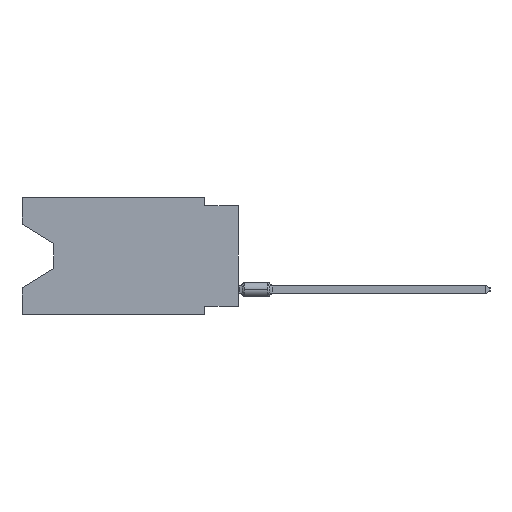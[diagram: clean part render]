
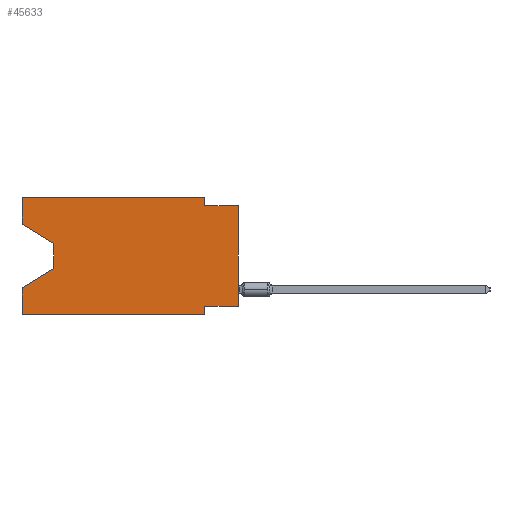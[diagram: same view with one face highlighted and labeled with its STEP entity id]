
A CAD part, left-side view. The second image highlights one B-rep face of the part: STEP entity #45633.
In plain terms, the highlighted planar face has unit normal (-1, 0, 0).
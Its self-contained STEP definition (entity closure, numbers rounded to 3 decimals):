
#1203 = LINE ( 'NONE', #77427, #64038 ) ;
#1259 = EDGE_CURVE ( 'NONE', #56919, #22937, #66565, .T. ) ;
#1292 = CARTESIAN_POINT ( 'NONE',  ( 0., 13.97, -3.505 ) ) ;
#2321 = CARTESIAN_POINT ( 'NONE',  ( 0., 2.54, -8.255 ) ) ;
#2335 = CARTESIAN_POINT ( 'NONE',  ( 0., 16.383, -2.038 ) ) ;
#3338 = CARTESIAN_POINT ( 'NONE',  ( 0., 16.383, -2.038 ) ) ;
#3871 = PLANE ( 'NONE',  #79965 ) ;
#4472 = LINE ( 'NONE', #100131, #5257 ) ;
#5257 = VECTOR ( 'NONE', #88839, 1000. ) ;
#7312 = CARTESIAN_POINT ( 'NONE',  ( 0., 13.97, -3.505 ) ) ;
#7677 = CARTESIAN_POINT ( 'NONE',  ( 0., 0., -8.255 ) ) ;
#10876 = EDGE_CURVE ( 'NONE', #61296, #36003, #45650, .T. ) ;
#11784 = VECTOR ( 'NONE', #57175, 1000. ) ;
#12044 = VECTOR ( 'NONE', #87257, 1000. ) ;
#12978 = VERTEX_POINT ( 'NONE', #103977 ) ;
#13083 = LINE ( 'NONE', #3338, #11784 ) ;
#14751 = VECTOR ( 'NONE', #19941, 1000. ) ;
#15023 = CARTESIAN_POINT ( 'NONE',  ( 0., 13.97, -5.385 ) ) ;
#15088 = EDGE_CURVE ( 'NONE', #56919, #23978, #79063, .T. ) ;
#15566 = CARTESIAN_POINT ( 'NONE',  ( 0., 0., 0. ) ) ;
#16709 = LINE ( 'NONE', #26407, #110979 ) ;
#16798 = CARTESIAN_POINT ( 'NONE',  ( 0., 2.54, -0.635 ) ) ;
#17405 = VECTOR ( 'NONE', #88220, 1000. ) ;
#17586 = EDGE_CURVE ( 'NONE', #28885, #36003, #4472, .T. ) ;
#19941 = DIRECTION ( 'NONE',  ( 0., 0., -1. ) ) ;
#21270 = VERTEX_POINT ( 'NONE', #2335 ) ;
#21811 = ORIENTED_EDGE ( 'NONE', *, *, #25461, .F. ) ;
#22937 = VERTEX_POINT ( 'NONE', #106627 ) ;
#23024 = CARTESIAN_POINT ( 'NONE',  ( 0., 2.54, 0. ) ) ;
#23466 = DIRECTION ( 'NONE',  ( 0., -1., 0. ) ) ;
#23978 = VERTEX_POINT ( 'NONE', #2321 ) ;
#24261 = DIRECTION ( 'NONE',  ( 0., 0., -1. ) ) ;
#24834 = LINE ( 'NONE', #94725, #79256 ) ;
#25461 = EDGE_CURVE ( 'NONE', #21270, #12978, #1203, .T. ) ;
#26407 = CARTESIAN_POINT ( 'NONE',  ( 0., 0., -0.635 ) ) ;
#28885 = VERTEX_POINT ( 'NONE', #103390 ) ;
#31616 = DIRECTION ( 'NONE',  ( 0., 0., 1. ) ) ;
#32459 = EDGE_CURVE ( 'NONE', #28885, #72429, #58411, .T. ) ;
#34808 = CARTESIAN_POINT ( 'NONE',  ( 0., 13.97, -5.385 ) ) ;
#36003 = VERTEX_POINT ( 'NONE', #92540 ) ;
#36623 = ORIENTED_EDGE ( 'NONE', *, *, #32459, .T. ) ;
#37901 = ORIENTED_EDGE ( 'NONE', *, *, #10876, .T. ) ;
#38016 = VERTEX_POINT ( 'NONE', #7312 ) ;
#38763 = ORIENTED_EDGE ( 'NONE', *, *, #107719, .T. ) ;
#43628 = DIRECTION ( 'NONE',  ( 0., 0., 1. ) ) ;
#45633 = ADVANCED_FACE ( 'NONE', ( #99533 ), #3871, .F. ) ;
#45650 = LINE ( 'NONE', #34808, #78965 ) ;
#56877 = EDGE_CURVE ( 'NONE', #12978, #84693, #59787, .T. ) ;
#56919 = VERTEX_POINT ( 'NONE', #7677 ) ;
#57175 = DIRECTION ( 'NONE',  ( 0., -0.855, -0.519 ) ) ;
#58200 = ORIENTED_EDGE ( 'NONE', *, *, #17586, .F. ) ;
#58411 = LINE ( 'NONE', #58966, #83168 ) ;
#58966 = CARTESIAN_POINT ( 'NONE',  ( 0., 16.383, -8.89 ) ) ;
#59787 = LINE ( 'NONE', #86138, #12044 ) ;
#61296 = VERTEX_POINT ( 'NONE', #15023 ) ;
#61596 = EDGE_LOOP ( 'NONE', ( #38763, #70685, #37901, #58200, #36623, #85194, #73847, #112691, #91731, #91290, #88924, #21811 ) ) ;
#61934 = EDGE_CURVE ( 'NONE', #84693, #83107, #82345, .T. ) ;
#64038 = VECTOR ( 'NONE', #43628, 1000. ) ;
#65166 = DIRECTION ( 'NONE',  ( 1., 0., 0. ) ) ;
#66565 = LINE ( 'NONE', #15566, #82760 ) ;
#70685 = ORIENTED_EDGE ( 'NONE', *, *, #84505, .T. ) ;
#71604 = CARTESIAN_POINT ( 'NONE',  ( 0., 0., -8.255 ) ) ;
#72429 = VERTEX_POINT ( 'NONE', #88360 ) ;
#73198 = CARTESIAN_POINT ( 'NONE',  ( 0., 2.54, 0. ) ) ;
#73847 = ORIENTED_EDGE ( 'NONE', *, *, #15088, .F. ) ;
#74050 = EDGE_CURVE ( 'NONE', #83107, #22937, #16709, .T. ) ;
#77427 = CARTESIAN_POINT ( 'NONE',  ( 0., 16.383, 0. ) ) ;
#78965 = VECTOR ( 'NONE', #88613, 1000. ) ;
#79063 = LINE ( 'NONE', #71604, #17405 ) ;
#79256 = VECTOR ( 'NONE', #24261, 1000. ) ;
#79965 = AXIS2_PLACEMENT_3D ( 'NONE', #108116, #65166, #100110 ) ;
#82345 = LINE ( 'NONE', #73198, #14751 ) ;
#82760 = VECTOR ( 'NONE', #31616, 1000. ) ;
#83107 = VERTEX_POINT ( 'NONE', #16798 ) ;
#83168 = VECTOR ( 'NONE', #23466, 1000. ) ;
#84315 = EDGE_CURVE ( 'NONE', #23978, #72429, #24834, .T. ) ;
#84505 = EDGE_CURVE ( 'NONE', #38016, #61296, #98085, .T. ) ;
#84693 = VERTEX_POINT ( 'NONE', #23024 ) ;
#85194 = ORIENTED_EDGE ( 'NONE', *, *, #84315, .F. ) ;
#86138 = CARTESIAN_POINT ( 'NONE',  ( 0., 16.383, 0. ) ) ;
#87124 = DIRECTION ( 'NONE',  ( 0., -1., 0. ) ) ;
#87257 = DIRECTION ( 'NONE',  ( 0., -1., 0. ) ) ;
#88220 = DIRECTION ( 'NONE',  ( 0., 1., 0. ) ) ;
#88353 = DIRECTION ( 'NONE',  ( 0., 0., -1. ) ) ;
#88360 = CARTESIAN_POINT ( 'NONE',  ( 0., 2.54, -8.89 ) ) ;
#88613 = DIRECTION ( 'NONE',  ( 0., 0.855, -0.519 ) ) ;
#88839 = DIRECTION ( 'NONE',  ( 0., 0., 1. ) ) ;
#88924 = ORIENTED_EDGE ( 'NONE', *, *, #56877, .F. ) ;
#91290 = ORIENTED_EDGE ( 'NONE', *, *, #61934, .F. ) ;
#91731 = ORIENTED_EDGE ( 'NONE', *, *, #74050, .F. ) ;
#92540 = CARTESIAN_POINT ( 'NONE',  ( 0., 16.383, -6.852 ) ) ;
#94725 = CARTESIAN_POINT ( 'NONE',  ( 0., 2.54, -8.89 ) ) ;
#98085 = LINE ( 'NONE', #1292, #112135 ) ;
#99533 = FACE_OUTER_BOUND ( 'NONE', #61596, .T. ) ;
#100110 = DIRECTION ( 'NONE',  ( 0., 0., -1. ) ) ;
#100131 = CARTESIAN_POINT ( 'NONE',  ( 0., 16.383, 0. ) ) ;
#103390 = CARTESIAN_POINT ( 'NONE',  ( 0., 16.383, -8.89 ) ) ;
#103977 = CARTESIAN_POINT ( 'NONE',  ( 0., 16.383, 0. ) ) ;
#106627 = CARTESIAN_POINT ( 'NONE',  ( 0., 0., -0.635 ) ) ;
#107719 = EDGE_CURVE ( 'NONE', #21270, #38016, #13083, .T. ) ;
#108116 = CARTESIAN_POINT ( 'NONE',  ( 0., 16.383, 0. ) ) ;
#110979 = VECTOR ( 'NONE', #87124, 1000. ) ;
#112135 = VECTOR ( 'NONE', #88353, 1000. ) ;
#112691 = ORIENTED_EDGE ( 'NONE', *, *, #1259, .T. ) ;
